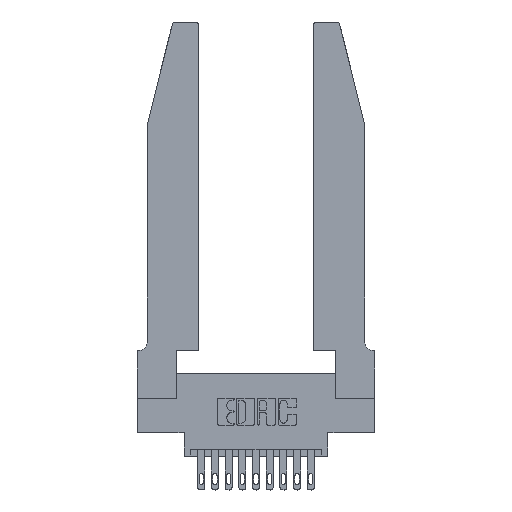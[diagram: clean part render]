
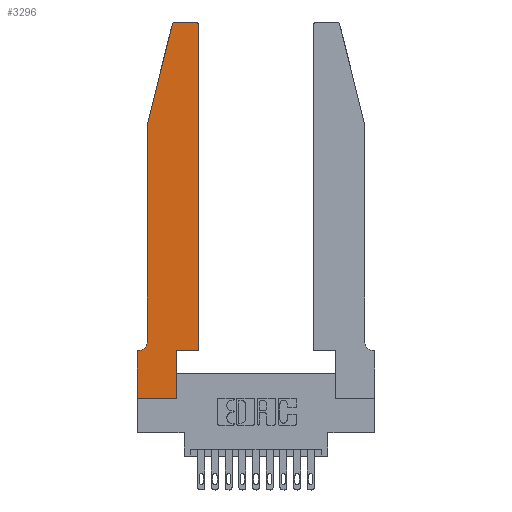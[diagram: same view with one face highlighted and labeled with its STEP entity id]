
A CAD part, top view. The second image highlights one B-rep face of the part: STEP entity #3296.
In plain terms, the highlighted planar face has unit normal (0, 0, 1).
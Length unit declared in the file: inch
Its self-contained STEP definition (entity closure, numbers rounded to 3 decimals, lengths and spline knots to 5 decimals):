
#76 = VERTEX_POINT ( 'NONE', #2064 ) ;
#298 = LINE ( 'NONE', #2591, #1668 ) ;
#301 = EDGE_CURVE ( 'NONE', #5199, #5900, #6575, .T. ) ;
#872 = EDGE_CURVE ( 'NONE', #10622, #6512, #10908, .T. ) ;
#1003 = CARTESIAN_POINT ( 'NONE',  ( 0., 0.35, 0.37 ) ) ;
#1201 = DIRECTION ( 'NONE',  ( 1., 0., 0. ) ) ;
#1309 = CARTESIAN_POINT ( 'NONE',  ( 0.284, 2.72, 0.37 ) ) ;
#1361 = DIRECTION ( 'NONE',  ( 1., 0., 0. ) ) ;
#1668 = VECTOR ( 'NONE', #11823, 39.37008 ) ;
#1693 = VERTEX_POINT ( 'NONE', #10006 ) ;
#1778 = EDGE_CURVE ( 'NONE', #6710, #8349, #9696, .T. ) ;
#2064 = CARTESIAN_POINT ( 'NONE',  ( 0.284, 2.75, 0.37 ) ) ;
#2382 = CARTESIAN_POINT ( 'NONE',  ( 0.4205, 2.72, 0.37 ) ) ;
#2524 = ORIENTED_EDGE ( 'NONE', *, *, #13394, .T. ) ;
#2541 = CARTESIAN_POINT ( 'NONE',  ( 0.0755, 0.35, 0.37 ) ) ;
#2591 = CARTESIAN_POINT ( 'NONE',  ( 0., 0., 0.37 ) ) ;
#2850 = ORIENTED_EDGE ( 'NONE', *, *, #8884, .T. ) ;
#3045 = AXIS2_PLACEMENT_3D ( 'NONE', #1309, #6331, #1201 ) ;
#3056 = ORIENTED_EDGE ( 'NONE', *, *, #9516, .T. ) ;
#3122 = CARTESIAN_POINT ( 'NONE',  ( 0.0755, 2., 0.37 ) ) ;
#3155 = CARTESIAN_POINT ( 'NONE',  ( 0., 0., 0.37 ) ) ;
#3206 = VECTOR ( 'NONE', #9172, 39.37008 ) ;
#3228 = LINE ( 'NONE', #3122, #14088 ) ;
#3288 = LINE ( 'NONE', #10121, #7426 ) ;
#3296 = ADVANCED_FACE ( 'NONE', ( #13182 ), #12517, .T. ) ;
#3377 = VERTEX_POINT ( 'NONE', #14125 ) ;
#3621 = LINE ( 'NONE', #13429, #15277 ) ;
#3689 = CARTESIAN_POINT ( 'NONE',  ( 0.2865, 0.35, 0.37 ) ) ;
#3732 = DIRECTION ( 'NONE',  ( 0., 0., -1. ) ) ;
#4029 = EDGE_CURVE ( 'NONE', #1693, #10622, #14362, .T. ) ;
#4535 = EDGE_CURVE ( 'NONE', #8349, #76, #3288, .T. ) ;
#4622 = EDGE_CURVE ( 'NONE', #6512, #16016, #12559, .T. ) ;
#5159 = ORIENTED_EDGE ( 'NONE', *, *, #8860, .T. ) ;
#5199 = VERTEX_POINT ( 'NONE', #8732 ) ;
#5224 = CARTESIAN_POINT ( 'NONE',  ( 0.0755, 0.42, 0.37 ) ) ;
#5498 = ORIENTED_EDGE ( 'NONE', *, *, #4535, .T. ) ;
#5609 = DIRECTION ( 'NONE',  ( -0.239, -0.971, 0. ) ) ;
#5648 = VECTOR ( 'NONE', #13786, 39.37008 ) ;
#5900 = VERTEX_POINT ( 'NONE', #5224 ) ;
#5956 = EDGE_CURVE ( 'NONE', #11197, #1693, #298, .T. ) ;
#6045 = AXIS2_PLACEMENT_3D ( 'NONE', #9975, #3732, #12547 ) ;
#6276 = AXIS2_PLACEMENT_3D ( 'NONE', #1003, #9939, #1361 ) ;
#6331 = DIRECTION ( 'NONE',  ( 0., 0., 1. ) ) ;
#6512 = VERTEX_POINT ( 'NONE', #15472 ) ;
#6575 = LINE ( 'NONE', #14060, #3206 ) ;
#6584 = VERTEX_POINT ( 'NONE', #13855 ) ;
#6619 = ORIENTED_EDGE ( 'NONE', *, *, #301, .T. ) ;
#6710 = VERTEX_POINT ( 'NONE', #14681 ) ;
#6813 = ORIENTED_EDGE ( 'NONE', *, *, #4029, .T. ) ;
#7104 = EDGE_CURVE ( 'NONE', #3377, #5199, #3228, .T. ) ;
#7426 = VECTOR ( 'NONE', #13501, 39.37008 ) ;
#7436 = DIRECTION ( 'NONE',  ( 1., 0., 0. ) ) ;
#7451 = CARTESIAN_POINT ( 'NONE',  ( 0.4205, 2.75, 0.37 ) ) ;
#8349 = VERTEX_POINT ( 'NONE', #7451 ) ;
#8382 = AXIS2_PLACEMENT_3D ( 'NONE', #2382, #9881, #7436 ) ;
#8435 = CARTESIAN_POINT ( 'NONE',  ( 0.4505, 0.35, 0.37 ) ) ;
#8664 = DIRECTION ( 'NONE',  ( 0., 1., 0. ) ) ;
#8732 = CARTESIAN_POINT ( 'NONE',  ( 0.0755, 2., 0.37 ) ) ;
#8860 = EDGE_CURVE ( 'NONE', #16016, #6710, #3621, .T. ) ;
#8867 = VECTOR ( 'NONE', #11974, 39.37008 ) ;
#8884 = EDGE_CURVE ( 'NONE', #6584, #11197, #13258, .T. ) ;
#9172 = DIRECTION ( 'NONE',  ( 0., -1., 0. ) ) ;
#9516 = EDGE_CURVE ( 'NONE', #76, #3377, #11284, .T. ) ;
#9696 = CIRCLE ( 'NONE', #8382, 0.03 ) ;
#9881 = DIRECTION ( 'NONE',  ( 0., 0., 1. ) ) ;
#9939 = DIRECTION ( 'NONE',  ( 0., 0., 1. ) ) ;
#9975 = CARTESIAN_POINT ( 'NONE',  ( 0.0055, 0.42, 0.37 ) ) ;
#10006 = CARTESIAN_POINT ( 'NONE',  ( 0., 0., 0.37 ) ) ;
#10121 = CARTESIAN_POINT ( 'NONE',  ( 0.2605, 2.75, 0.37 ) ) ;
#10224 = ORIENTED_EDGE ( 'NONE', *, *, #5956, .T. ) ;
#10622 = VERTEX_POINT ( 'NONE', #13766 ) ;
#10908 = LINE ( 'NONE', #3689, #15638 ) ;
#10930 = VECTOR ( 'NONE', #11240, 39.37008 ) ;
#10977 = DIRECTION ( 'NONE',  ( 0., 1., 0. ) ) ;
#11188 = ORIENTED_EDGE ( 'NONE', *, *, #7104, .T. ) ;
#11197 = VERTEX_POINT ( 'NONE', #12712 ) ;
#11240 = DIRECTION ( 'NONE',  ( -1., 0., 0. ) ) ;
#11284 = CIRCLE ( 'NONE', #3045, 0.03 ) ;
#11823 = DIRECTION ( 'NONE',  ( 0., -1., 0. ) ) ;
#11974 = DIRECTION ( 'NONE',  ( 1., 0., 0. ) ) ;
#12375 = ORIENTED_EDGE ( 'NONE', *, *, #872, .T. ) ;
#12517 = PLANE ( 'NONE',  #6276 ) ;
#12547 = DIRECTION ( 'NONE',  ( -1., 0., 0. ) ) ;
#12559 = LINE ( 'NONE', #15028, #5648 ) ;
#12712 = CARTESIAN_POINT ( 'NONE',  ( 0., 0.35, 0.37 ) ) ;
#12761 = CIRCLE ( 'NONE', #6045, 0.07 ) ;
#13182 = FACE_OUTER_BOUND ( 'NONE', #15880, .T. ) ;
#13258 = LINE ( 'NONE', #2541, #10930 ) ;
#13394 = EDGE_CURVE ( 'NONE', #5900, #6584, #12761, .T. ) ;
#13429 = CARTESIAN_POINT ( 'NONE',  ( 0.4505, 0.35, 0.37 ) ) ;
#13486 = ORIENTED_EDGE ( 'NONE', *, *, #4622, .T. ) ;
#13501 = DIRECTION ( 'NONE',  ( -1., 0., 0. ) ) ;
#13766 = CARTESIAN_POINT ( 'NONE',  ( 0.2865, 0., 0.37 ) ) ;
#13786 = DIRECTION ( 'NONE',  ( 1., 0., 0. ) ) ;
#13855 = CARTESIAN_POINT ( 'NONE',  ( 0.0055, 0.35, 0.37 ) ) ;
#14060 = CARTESIAN_POINT ( 'NONE',  ( 0.0755, 2., 0.37 ) ) ;
#14088 = VECTOR ( 'NONE', #5609, 39.37008 ) ;
#14125 = CARTESIAN_POINT ( 'NONE',  ( 0.25487, 2.72718, 0.37 ) ) ;
#14362 = LINE ( 'NONE', #3155, #8867 ) ;
#14681 = CARTESIAN_POINT ( 'NONE',  ( 0.4505, 2.72, 0.37 ) ) ;
#15028 = CARTESIAN_POINT ( 'NONE',  ( 0.4505, 0.35, 0.37 ) ) ;
#15277 = VECTOR ( 'NONE', #10977, 39.37008 ) ;
#15472 = CARTESIAN_POINT ( 'NONE',  ( 0.2865, 0.35, 0.37 ) ) ;
#15638 = VECTOR ( 'NONE', #8664, 39.37008 ) ;
#15880 = EDGE_LOOP ( 'NONE', ( #5498, #3056, #11188, #6619, #2524, #2850, #10224, #6813, #12375, #13486, #5159, #16198 ) ) ;
#16016 = VERTEX_POINT ( 'NONE', #8435 ) ;
#16198 = ORIENTED_EDGE ( 'NONE', *, *, #1778, .T. ) ;
